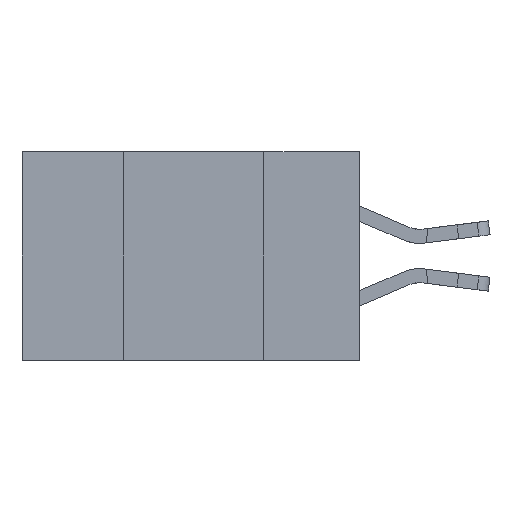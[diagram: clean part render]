
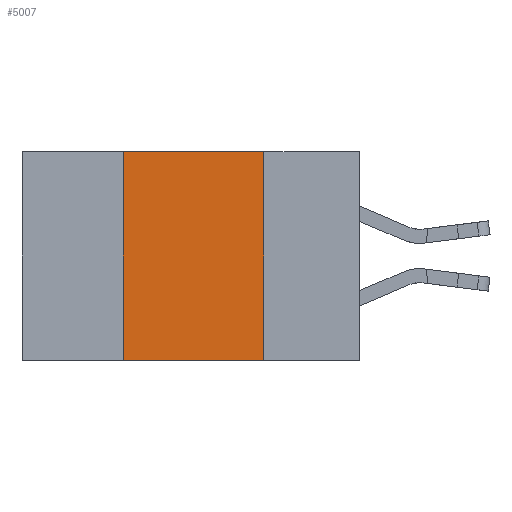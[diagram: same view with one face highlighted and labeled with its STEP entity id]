
A CAD part, left-side view. The second image highlights one B-rep face of the part: STEP entity #5007.
In plain terms, the highlighted planar face has unit normal (-1, 0, 0).
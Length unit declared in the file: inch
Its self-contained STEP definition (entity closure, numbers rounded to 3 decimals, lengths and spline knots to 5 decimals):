
#162 = ORIENTED_EDGE ( 'NONE', *, *, #6189, .F. ) ;
#278 = DIRECTION ( 'NONE',  ( 0., 0., -1. ) ) ;
#989 = EDGE_CURVE ( 'NONE', #24991, #9483, #12663, .T. ) ;
#1333 = VECTOR ( 'NONE', #278, 39.37008 ) ;
#2747 = CARTESIAN_POINT ( 'NONE',  ( 0., 0.17, 0. ) ) ;
#3310 = EDGE_CURVE ( 'NONE', #8090, #9483, #7504, .T. ) ;
#3453 = LINE ( 'NONE', #19819, #19370 ) ;
#3974 = LINE ( 'NONE', #24689, #8835 ) ;
#5007 = ADVANCED_FACE ( 'NONE', ( #25319 ), #15884, .F. ) ;
#5275 = CARTESIAN_POINT ( 'NONE',  ( 0., 0.17, -0.37 ) ) ;
#6189 = EDGE_CURVE ( 'NONE', #13207, #8090, #3453, .T. ) ;
#6241 = DIRECTION ( 'NONE',  ( 0., -1., 0. ) ) ;
#7504 = LINE ( 'NONE', #19241, #1333 ) ;
#8090 = VERTEX_POINT ( 'NONE', #2747 ) ;
#8835 = VECTOR ( 'NONE', #10244, 39.37008 ) ;
#9160 = DIRECTION ( 'NONE',  ( 0., 0., -1. ) ) ;
#9483 = VERTEX_POINT ( 'NONE', #5275 ) ;
#9917 = ORIENTED_EDGE ( 'NONE', *, *, #25406, .F. ) ;
#10244 = DIRECTION ( 'NONE',  ( 0., 0., 1. ) ) ;
#11677 = VECTOR ( 'NONE', #6241, 39.37008 ) ;
#12663 = LINE ( 'NONE', #18966, #11677 ) ;
#13207 = VERTEX_POINT ( 'NONE', #21912 ) ;
#13833 = ORIENTED_EDGE ( 'NONE', *, *, #3310, .F. ) ;
#15884 = PLANE ( 'NONE',  #20372 ) ;
#17231 = ORIENTED_EDGE ( 'NONE', *, *, #989, .T. ) ;
#17766 = CARTESIAN_POINT ( 'NONE',  ( 0., 0.42, -0.37 ) ) ;
#17907 = DIRECTION ( 'NONE',  ( 0., -1., 0. ) ) ;
#18966 = CARTESIAN_POINT ( 'NONE',  ( 0., 0.6, -0.37 ) ) ;
#19241 = CARTESIAN_POINT ( 'NONE',  ( 0., 0.17, 0. ) ) ;
#19370 = VECTOR ( 'NONE', #17907, 39.37008 ) ;
#19819 = CARTESIAN_POINT ( 'NONE',  ( 0., 0.6, 0. ) ) ;
#20372 = AXIS2_PLACEMENT_3D ( 'NONE', #24915, #24093, #9160 ) ;
#20864 = EDGE_LOOP ( 'NONE', ( #13833, #162, #9917, #17231 ) ) ;
#21912 = CARTESIAN_POINT ( 'NONE',  ( 0., 0.42, 0. ) ) ;
#24093 = DIRECTION ( 'NONE',  ( 1., 0., 0. ) ) ;
#24689 = CARTESIAN_POINT ( 'NONE',  ( 0., 0.42, 0. ) ) ;
#24915 = CARTESIAN_POINT ( 'NONE',  ( 0., 0.6, 0. ) ) ;
#24991 = VERTEX_POINT ( 'NONE', #17766 ) ;
#25319 = FACE_OUTER_BOUND ( 'NONE', #20864, .T. ) ;
#25406 = EDGE_CURVE ( 'NONE', #24991, #13207, #3974, .T. ) ;
